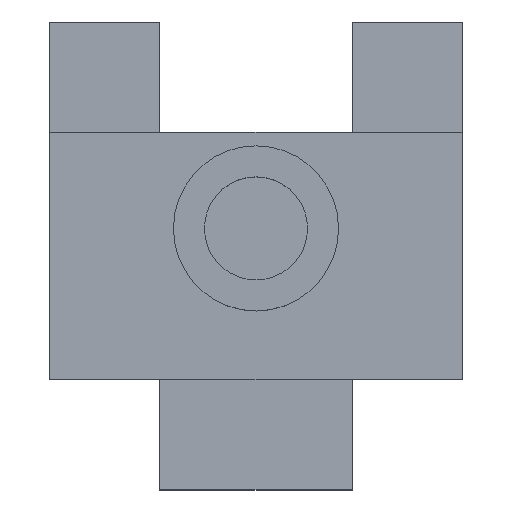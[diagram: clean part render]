
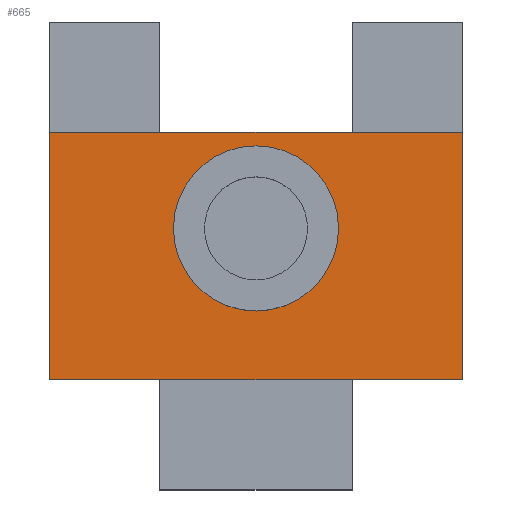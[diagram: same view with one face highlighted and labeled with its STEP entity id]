
A CAD part, top view. The second image highlights one B-rep face of the part: STEP entity #665.
In plain terms, the highlighted planar face has unit normal (0, 0, 1).
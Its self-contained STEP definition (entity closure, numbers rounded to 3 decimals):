
#1 = CARTESIAN_POINT ( 'NONE',  ( 65.625, 25.104, -203.587 ) ) ;
#4 = CARTESIAN_POINT ( 'NONE',  ( 65.625, 116.84, -203.587 ) ) ;
#28 = AXIS2_PLACEMENT_3D ( 'NONE', #622, #715, #1074 ) ;
#30 = DIRECTION ( 'NONE',  ( 0., -1., 0. ) ) ;
#33 = EDGE_CURVE ( 'NONE', #1065, #951, #936, .T. ) ;
#41 = CARTESIAN_POINT ( 'NONE',  ( 48.75, 103.715, -203.587 ) ) ;
#54 = CARTESIAN_POINT ( 'NONE',  ( 9.375, 116.84, -203.587 ) ) ;
#55 = DIRECTION ( 'NONE',  ( -1., 0., 0. ) ) ;
#65 = DIRECTION ( 'NONE',  ( 0., 0., -1. ) ) ;
#91 = EDGE_CURVE ( 'NONE', #143, #493, #885, .T. ) ;
#94 = EDGE_LOOP ( 'NONE', ( #1091, #750, #977, #623, #225, #782, #199, #439 ) ) ;
#100 = DIRECTION ( 'NONE',  ( -1., 0., 0. ) ) ;
#113 = CARTESIAN_POINT ( 'NONE',  ( 9.375, 116.84, -203.587 ) ) ;
#130 = VERTEX_POINT ( 'NONE', #54 ) ;
#134 = PLANE ( 'NONE',  #988 ) ;
#142 = CARTESIAN_POINT ( 'NONE',  ( 65.625, 83.09, -203.587 ) ) ;
#143 = VERTEX_POINT ( 'NONE', #830 ) ;
#151 = CARTESIAN_POINT ( 'NONE',  ( 50.625, 116.84, -203.587 ) ) ;
#162 = CARTESIAN_POINT ( 'NONE',  ( 65.625, 83.09, -203.587 ) ) ;
#175 = EDGE_CURVE ( 'NONE', #1086, #900, #838, .T. ) ;
#180 = CIRCLE ( 'NONE', #28, 11.25 ) ;
#199 = ORIENTED_EDGE ( 'NONE', *, *, #1008, .F. ) ;
#206 = VERTEX_POINT ( 'NONE', #966 ) ;
#222 = DIRECTION ( 'NONE',  ( -1., 0., 0. ) ) ;
#225 = ORIENTED_EDGE ( 'NONE', *, *, #1036, .T. ) ;
#236 = DIRECTION ( 'NONE',  ( -1., 0., 0. ) ) ;
#238 = DIRECTION ( 'NONE',  ( -1., 0., 0. ) ) ;
#249 = CARTESIAN_POINT ( 'NONE',  ( 65.625, 83.09, -203.587 ) ) ;
#255 = ORIENTED_EDGE ( 'NONE', *, *, #91, .F. ) ;
#275 = CARTESIAN_POINT ( 'NONE',  ( 24.375, 83.09, -203.587 ) ) ;
#313 = CARTESIAN_POINT ( 'NONE',  ( 65.625, 116.84, -203.587 ) ) ;
#316 = DIRECTION ( 'NONE',  ( -1., 0., 0. ) ) ;
#351 = DIRECTION ( 'NONE',  ( 0., 1., 0. ) ) ;
#400 = CARTESIAN_POINT ( 'NONE',  ( 65.625, 116.84, -203.587 ) ) ;
#439 = ORIENTED_EDGE ( 'NONE', *, *, #33, .F. ) ;
#449 = DIRECTION ( 'NONE',  ( 0., 0., 1. ) ) ;
#454 = VECTOR ( 'NONE', #351, 1000. ) ;
#458 = LINE ( 'NONE', #1, #454 ) ;
#473 = LINE ( 'NONE', #113, #662 ) ;
#490 = VECTOR ( 'NONE', #236, 1000. ) ;
#493 = VERTEX_POINT ( 'NONE', #41 ) ;
#494 = LINE ( 'NONE', #162, #490 ) ;
#517 = VECTOR ( 'NONE', #1053, 1000. ) ;
#520 = LINE ( 'NONE', #4, #517 ) ;
#599 = EDGE_CURVE ( 'NONE', #493, #143, #180, .T. ) ;
#604 = VECTOR ( 'NONE', #316, 1000. ) ;
#609 = LINE ( 'NONE', #400, #604 ) ;
#620 = LINE ( 'NONE', #1088, #644 ) ;
#622 = CARTESIAN_POINT ( 'NONE',  ( 37.5, 103.715, -203.587 ) ) ;
#623 = ORIENTED_EDGE ( 'NONE', *, *, #950, .T. ) ;
#632 = FACE_BOUND ( 'NONE', #730, .T. ) ;
#635 = FACE_OUTER_BOUND ( 'NONE', #94, .T. ) ;
#644 = VECTOR ( 'NONE', #222, 1000. ) ;
#662 = VECTOR ( 'NONE', #30, 1000. ) ;
#665 = ADVANCED_FACE ( 'NONE', ( #635, #632 ), #134, .F. ) ;
#673 = EDGE_CURVE ( 'NONE', #1089, #206, #620, .T. ) ;
#691 = EDGE_CURVE ( 'NONE', #900, #694, #609, .T. ) ;
#694 = VERTEX_POINT ( 'NONE', #985 ) ;
#715 = DIRECTION ( 'NONE',  ( 0., 0., 1. ) ) ;
#716 = CARTESIAN_POINT ( 'NONE',  ( 65.625, 116.84, -203.587 ) ) ;
#730 = EDGE_LOOP ( 'NONE', ( #255, #873 ) ) ;
#750 = ORIENTED_EDGE ( 'NONE', *, *, #175, .T. ) ;
#782 = ORIENTED_EDGE ( 'NONE', *, *, #673, .F. ) ;
#830 = CARTESIAN_POINT ( 'NONE',  ( 26.25, 103.715, -203.587 ) ) ;
#838 = LINE ( 'NONE', #983, #841 ) ;
#841 = VECTOR ( 'NONE', #238, 1000. ) ;
#847 = AXIS2_PLACEMENT_3D ( 'NONE', #952, #449, #1020 ) ;
#873 = ORIENTED_EDGE ( 'NONE', *, *, #599, .F. ) ;
#885 = CIRCLE ( 'NONE', #847, 11.25 ) ;
#900 = VERTEX_POINT ( 'NONE', #151 ) ;
#928 = VECTOR ( 'NONE', #100, 1000. ) ;
#933 = CARTESIAN_POINT ( 'NONE',  ( 50.625, 83.09, -203.587 ) ) ;
#936 = LINE ( 'NONE', #142, #928 ) ;
#950 = EDGE_CURVE ( 'NONE', #694, #130, #520, .T. ) ;
#951 = VERTEX_POINT ( 'NONE', #933 ) ;
#952 = CARTESIAN_POINT ( 'NONE',  ( 37.5, 103.715, -203.587 ) ) ;
#966 = CARTESIAN_POINT ( 'NONE',  ( 9.375, 83.09, -203.587 ) ) ;
#977 = ORIENTED_EDGE ( 'NONE', *, *, #691, .T. ) ;
#983 = CARTESIAN_POINT ( 'NONE',  ( 65.625, 116.84, -203.587 ) ) ;
#985 = CARTESIAN_POINT ( 'NONE',  ( 24.375, 116.84, -203.587 ) ) ;
#988 = AXIS2_PLACEMENT_3D ( 'NONE', #716, #65, #55 ) ;
#1008 = EDGE_CURVE ( 'NONE', #951, #1089, #494, .T. ) ;
#1020 = DIRECTION ( 'NONE',  ( -1., 0., 0. ) ) ;
#1036 = EDGE_CURVE ( 'NONE', #130, #206, #473, .T. ) ;
#1053 = DIRECTION ( 'NONE',  ( -1., 0., 0. ) ) ;
#1065 = VERTEX_POINT ( 'NONE', #249 ) ;
#1074 = DIRECTION ( 'NONE',  ( -1., 0., 0. ) ) ;
#1086 = VERTEX_POINT ( 'NONE', #313 ) ;
#1088 = CARTESIAN_POINT ( 'NONE',  ( 65.625, 83.09, -203.587 ) ) ;
#1089 = VERTEX_POINT ( 'NONE', #275 ) ;
#1091 = ORIENTED_EDGE ( 'NONE', *, *, #1099, .T. ) ;
#1099 = EDGE_CURVE ( 'NONE', #1065, #1086, #458, .T. ) ;
